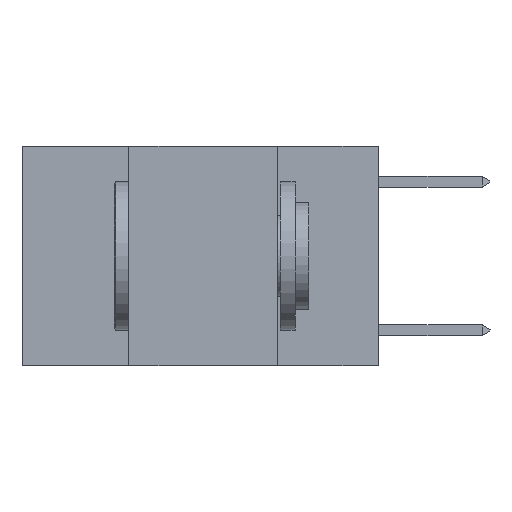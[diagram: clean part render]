
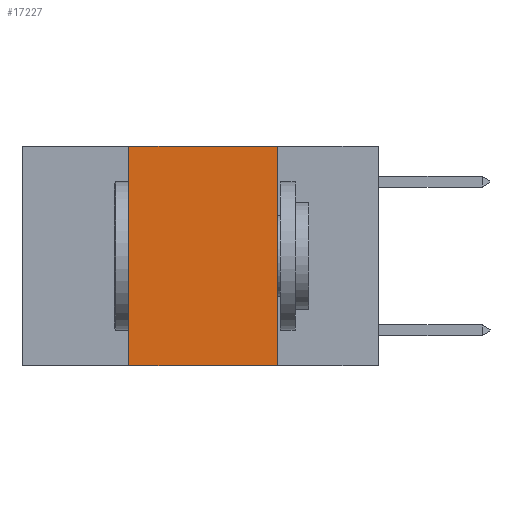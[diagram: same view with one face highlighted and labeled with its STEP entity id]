
A CAD part, left-side view. The second image highlights one B-rep face of the part: STEP entity #17227.
In plain terms, the highlighted planar face has unit normal (-1, 0, 0).
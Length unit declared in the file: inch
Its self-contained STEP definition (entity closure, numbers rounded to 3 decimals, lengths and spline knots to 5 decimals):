
#147 = EDGE_CURVE ( 'NONE', #5872, #2434, #21636, .T. ) ;
#290 = CARTESIAN_POINT ( 'NONE',  ( 0., 0.42, -0.37 ) ) ;
#2327 = EDGE_LOOP ( 'NONE', ( #5636, #14457, #13072, #18498 ) ) ;
#2411 = CARTESIAN_POINT ( 'NONE',  ( 0., 0.6, 0. ) ) ;
#2434 = VERTEX_POINT ( 'NONE', #12511 ) ;
#2502 = DIRECTION ( 'NONE',  ( 0., -1., 0. ) ) ;
#2919 = DIRECTION ( 'NONE',  ( 0., 0., -1. ) ) ;
#3034 = CARTESIAN_POINT ( 'NONE',  ( 0., 0.17, 0. ) ) ;
#5073 = EDGE_CURVE ( 'NONE', #14329, #15651, #14584, .T. ) ;
#5279 = EDGE_CURVE ( 'NONE', #5872, #14329, #13338, .T. ) ;
#5614 = PLANE ( 'NONE',  #12701 ) ;
#5636 = ORIENTED_EDGE ( 'NONE', *, *, #11161, .F. ) ;
#5872 = VERTEX_POINT ( 'NONE', #290 ) ;
#7454 = DIRECTION ( 'NONE',  ( 0., 0., -1. ) ) ;
#8834 = FACE_OUTER_BOUND ( 'NONE', #2327, .T. ) ;
#10082 = CARTESIAN_POINT ( 'NONE',  ( 0., 0.42, 0. ) ) ;
#11161 = EDGE_CURVE ( 'NONE', #15651, #2434, #19179, .T. ) ;
#12511 = CARTESIAN_POINT ( 'NONE',  ( 0., 0.17, -0.37 ) ) ;
#12701 = AXIS2_PLACEMENT_3D ( 'NONE', #16027, #17661, #7454 ) ;
#12990 = VECTOR ( 'NONE', #20652, 39.37008 ) ;
#13072 = ORIENTED_EDGE ( 'NONE', *, *, #5279, .F. ) ;
#13338 = LINE ( 'NONE', #20719, #12990 ) ;
#14300 = VECTOR ( 'NONE', #2502, 39.37008 ) ;
#14329 = VERTEX_POINT ( 'NONE', #10082 ) ;
#14457 = ORIENTED_EDGE ( 'NONE', *, *, #5073, .F. ) ;
#14584 = LINE ( 'NONE', #2411, #14300 ) ;
#14918 = DIRECTION ( 'NONE',  ( 0., -1., 0. ) ) ;
#15651 = VERTEX_POINT ( 'NONE', #17033 ) ;
#15723 = CARTESIAN_POINT ( 'NONE',  ( 0., 0.6, -0.37 ) ) ;
#16027 = CARTESIAN_POINT ( 'NONE',  ( 0., 0.6, 0. ) ) ;
#17033 = CARTESIAN_POINT ( 'NONE',  ( 0., 0.17, 0. ) ) ;
#17227 = ADVANCED_FACE ( 'NONE', ( #8834 ), #5614, .F. ) ;
#17661 = DIRECTION ( 'NONE',  ( 1., 0., 0. ) ) ;
#18498 = ORIENTED_EDGE ( 'NONE', *, *, #147, .T. ) ;
#19018 = VECTOR ( 'NONE', #2919, 39.37008 ) ;
#19179 = LINE ( 'NONE', #3034, #19018 ) ;
#20652 = DIRECTION ( 'NONE',  ( 0., 0., 1. ) ) ;
#20719 = CARTESIAN_POINT ( 'NONE',  ( 0., 0.42, 0. ) ) ;
#21577 = VECTOR ( 'NONE', #14918, 39.37008 ) ;
#21636 = LINE ( 'NONE', #15723, #21577 ) ;
